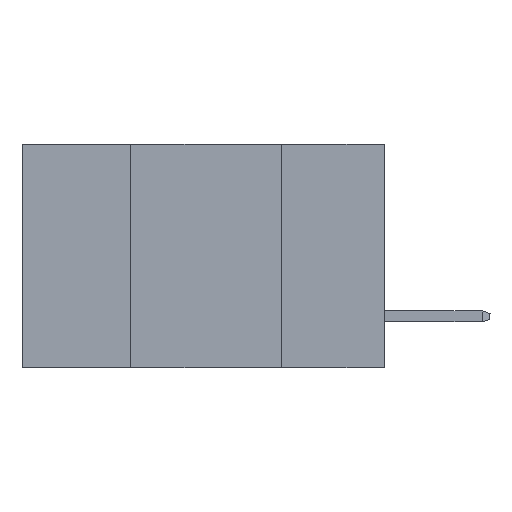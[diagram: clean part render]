
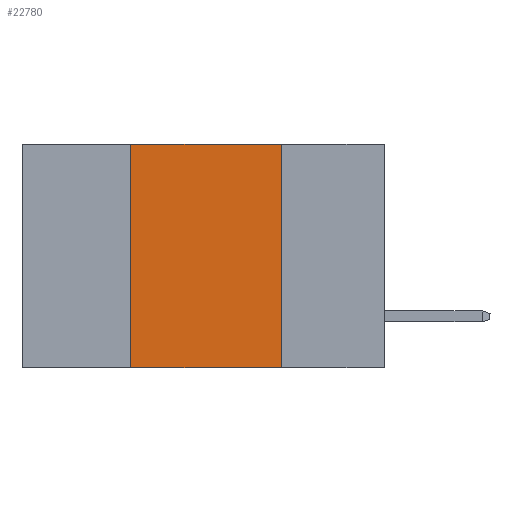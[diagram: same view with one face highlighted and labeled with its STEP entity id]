
A CAD part, left-side view. The second image highlights one B-rep face of the part: STEP entity #22780.
In plain terms, the highlighted planar face has unit normal (-1, 0, 0).
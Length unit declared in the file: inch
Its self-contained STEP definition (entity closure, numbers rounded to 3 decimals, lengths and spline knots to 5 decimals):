
#129 = DIRECTION ( 'NONE',  ( 0., -1., 0. ) ) ;
#501 = CARTESIAN_POINT ( 'NONE',  ( 0., 0.17, -0.37 ) ) ;
#966 = VERTEX_POINT ( 'NONE', #11178 ) ;
#1765 = CARTESIAN_POINT ( 'NONE',  ( 0., 0.17, -0.37 ) ) ;
#2599 = FACE_OUTER_BOUND ( 'NONE', #8123, .T. ) ;
#3213 = DIRECTION ( 'NONE',  ( 0., 0., -1. ) ) ;
#3955 = CARTESIAN_POINT ( 'NONE',  ( 0., 0.6, -0.37 ) ) ;
#4059 = DIRECTION ( 'NONE',  ( 0., 0., -1. ) ) ;
#5080 = DIRECTION ( 'NONE',  ( 0., 0., 1. ) ) ;
#5254 = DIRECTION ( 'NONE',  ( 1., 0., 0. ) ) ;
#5498 = LINE ( 'NONE', #17576, #22211 ) ;
#6253 = ORIENTED_EDGE ( 'NONE', *, *, #9503, .F. ) ;
#6986 = VECTOR ( 'NONE', #4059, 39.37008 ) ;
#7514 = EDGE_CURVE ( 'NONE', #8257, #10524, #5498, .T. ) ;
#8123 = EDGE_LOOP ( 'NONE', ( #18431, #13488, #6253, #15467 ) ) ;
#8140 = CARTESIAN_POINT ( 'NONE',  ( 0., 0.17, 0. ) ) ;
#8257 = VERTEX_POINT ( 'NONE', #17741 ) ;
#9266 = AXIS2_PLACEMENT_3D ( 'NONE', #18136, #5254, #3213 ) ;
#9503 = EDGE_CURVE ( 'NONE', #966, #8257, #14498, .T. ) ;
#10524 = VERTEX_POINT ( 'NONE', #8140 ) ;
#11178 = CARTESIAN_POINT ( 'NONE',  ( 0., 0.42, -0.37 ) ) ;
#11318 = LINE ( 'NONE', #1765, #6986 ) ;
#11717 = DIRECTION ( 'NONE',  ( 0., -1., 0. ) ) ;
#12061 = EDGE_CURVE ( 'NONE', #10524, #18363, #11318, .T. ) ;
#12069 = VECTOR ( 'NONE', #5080, 39.37008 ) ;
#13488 = ORIENTED_EDGE ( 'NONE', *, *, #7514, .F. ) ;
#14498 = LINE ( 'NONE', #16780, #12069 ) ;
#15467 = ORIENTED_EDGE ( 'NONE', *, *, #23006, .T. ) ;
#16780 = CARTESIAN_POINT ( 'NONE',  ( 0., 0.42, -0.37 ) ) ;
#17576 = CARTESIAN_POINT ( 'NONE',  ( 0., 0.6, 0. ) ) ;
#17741 = CARTESIAN_POINT ( 'NONE',  ( 0., 0.42, 0. ) ) ;
#18136 = CARTESIAN_POINT ( 'NONE',  ( 0., 0.6, 0. ) ) ;
#18266 = PLANE ( 'NONE',  #9266 ) ;
#18363 = VERTEX_POINT ( 'NONE', #501 ) ;
#18431 = ORIENTED_EDGE ( 'NONE', *, *, #12061, .F. ) ;
#21384 = LINE ( 'NONE', #3955, #21856 ) ;
#21856 = VECTOR ( 'NONE', #11717, 39.37008 ) ;
#22211 = VECTOR ( 'NONE', #129, 39.37008 ) ;
#22780 = ADVANCED_FACE ( 'NONE', ( #2599 ), #18266, .F. ) ;
#23006 = EDGE_CURVE ( 'NONE', #966, #18363, #21384, .T. ) ;
